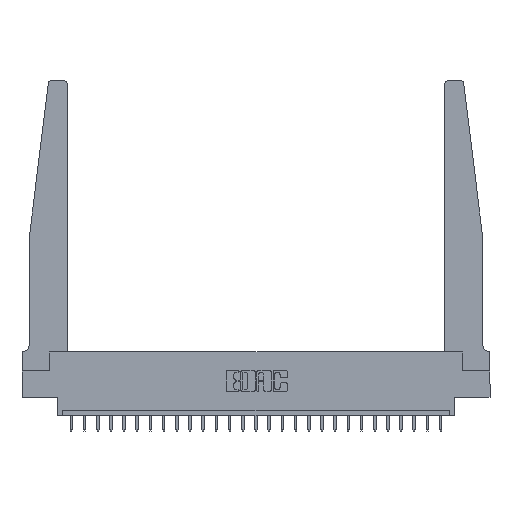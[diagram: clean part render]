
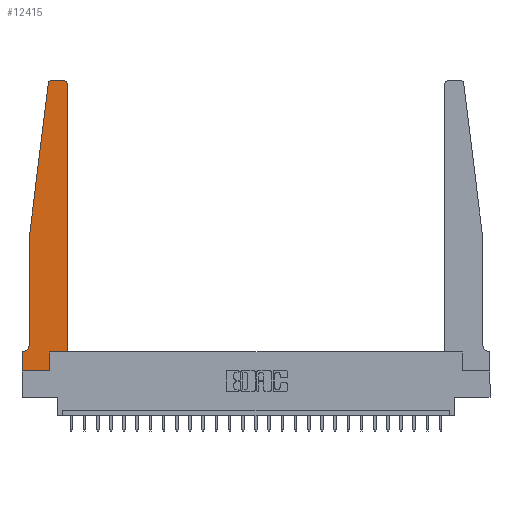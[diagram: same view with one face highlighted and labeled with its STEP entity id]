
A CAD part, top view. The second image highlights one B-rep face of the part: STEP entity #12415.
In plain terms, the highlighted planar face has unit normal (0, 0, 1).
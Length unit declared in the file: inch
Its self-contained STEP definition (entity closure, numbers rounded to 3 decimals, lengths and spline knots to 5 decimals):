
#265 = CARTESIAN_POINT ( 'NONE',  ( 0.27653, 2.75, 0.37 ) ) ;
#551 = VERTEX_POINT ( 'NONE', #13449 ) ;
#1065 = CIRCLE ( 'NONE', #18490, 0.03 ) ;
#1085 = EDGE_CURVE ( 'NONE', #22084, #10437, #18682, .T. ) ;
#1307 = CARTESIAN_POINT ( 'NONE',  ( 0.065, 1.25, 0.37 ) ) ;
#1937 = ORIENTED_EDGE ( 'NONE', *, *, #7434, .T. ) ;
#2708 = FACE_OUTER_BOUND ( 'NONE', #15776, .T. ) ;
#2877 = VERTEX_POINT ( 'NONE', #5473 ) ;
#2949 = VERTEX_POINT ( 'NONE', #265 ) ;
#3255 = ORIENTED_EDGE ( 'NONE', *, *, #1085, .T. ) ;
#3620 = DIRECTION ( 'NONE',  ( 1., 0., 0. ) ) ;
#3899 = DIRECTION ( 'NONE',  ( -1., 0., 0. ) ) ;
#4337 = ORIENTED_EDGE ( 'NONE', *, *, #23094, .T. ) ;
#4642 = VECTOR ( 'NONE', #22095, 39.37008 ) ;
#4856 = CARTESIAN_POINT ( 'NONE',  ( 0., 0.1875, 0.37 ) ) ;
#4949 = VECTOR ( 'NONE', #19105, 39.37008 ) ;
#5077 = LINE ( 'NONE', #8885, #6246 ) ;
#5325 = ORIENTED_EDGE ( 'NONE', *, *, #13525, .T. ) ;
#5349 = EDGE_CURVE ( 'NONE', #2949, #21349, #1065, .T. ) ;
#5393 = CARTESIAN_POINT ( 'NONE',  ( 0.27653, 2.72, 0.37 ) ) ;
#5473 = CARTESIAN_POINT ( 'NONE',  ( 0.015, 0.1875, 0.37 ) ) ;
#5707 = VECTOR ( 'NONE', #24729, 39.37008 ) ;
#5776 = CARTESIAN_POINT ( 'NONE',  ( 0.065, 1.25, 0.37 ) ) ;
#5852 = VERTEX_POINT ( 'NONE', #11840 ) ;
#6006 = ORIENTED_EDGE ( 'NONE', *, *, #8162, .T. ) ;
#6246 = VECTOR ( 'NONE', #9011, 39.37008 ) ;
#6573 = VECTOR ( 'NONE', #14024, 39.37008 ) ;
#7024 = CIRCLE ( 'NONE', #11896, 0.05 ) ;
#7296 = DIRECTION ( 'NONE',  ( 0., 0., 1. ) ) ;
#7434 = EDGE_CURVE ( 'NONE', #551, #16910, #12956, .T. ) ;
#7907 = CIRCLE ( 'NONE', #13582, 0.03 ) ;
#7951 = LINE ( 'NONE', #21270, #11808 ) ;
#8162 = EDGE_CURVE ( 'NONE', #11863, #20647, #7907, .T. ) ;
#8324 = CARTESIAN_POINT ( 'NONE',  ( 0.425, 2.72, 0.37 ) ) ;
#8431 = VECTOR ( 'NONE', #19429, 39.37008 ) ;
#8752 = CARTESIAN_POINT ( 'NONE',  ( 0.425, 0.18, 0.37 ) ) ;
#8885 = CARTESIAN_POINT ( 'NONE',  ( 0.25, 2.75, 0.37 ) ) ;
#9011 = DIRECTION ( 'NONE',  ( -1., 0., 0. ) ) ;
#9510 = CARTESIAN_POINT ( 'NONE',  ( 0.425, 0.18, 0.37 ) ) ;
#9740 = CARTESIAN_POINT ( 'NONE',  ( 0.395, 2.75, 0.37 ) ) ;
#9754 = DIRECTION ( 'NONE',  ( 0., 0., -1. ) ) ;
#9879 = CARTESIAN_POINT ( 'NONE',  ( 0.015, 0.2375, 0.37 ) ) ;
#10157 = CARTESIAN_POINT ( 'NONE',  ( 0.425, 0.18, 0.37 ) ) ;
#10437 = VERTEX_POINT ( 'NONE', #24971 ) ;
#10454 = DIRECTION ( 'NONE',  ( 0., 0., 1. ) ) ;
#10703 = PLANE ( 'NONE',  #14245 ) ;
#11179 = ORIENTED_EDGE ( 'NONE', *, *, #24212, .T. ) ;
#11567 = ORIENTED_EDGE ( 'NONE', *, *, #13350, .T. ) ;
#11808 = VECTOR ( 'NONE', #3899, 39.37008 ) ;
#11840 = CARTESIAN_POINT ( 'NONE',  ( 0., 0.1875, 0.37 ) ) ;
#11863 = VERTEX_POINT ( 'NONE', #8324 ) ;
#11896 = AXIS2_PLACEMENT_3D ( 'NONE', #9879, #9754, #17480 ) ;
#12007 = LINE ( 'NONE', #5776, #6573 ) ;
#12317 = VERTEX_POINT ( 'NONE', #16888 ) ;
#12415 = ADVANCED_FACE ( 'NONE', ( #2708 ), #10703, .T. ) ;
#12926 = LINE ( 'NONE', #9510, #5707 ) ;
#12956 = LINE ( 'NONE', #10157, #8431 ) ;
#13350 = EDGE_CURVE ( 'NONE', #5852, #12317, #22928, .T. ) ;
#13364 = LINE ( 'NONE', #17874, #24328 ) ;
#13449 = CARTESIAN_POINT ( 'NONE',  ( 0.2605, 0.18, 0.37 ) ) ;
#13525 = EDGE_CURVE ( 'NONE', #21349, #22084, #12007, .T. ) ;
#13582 = AXIS2_PLACEMENT_3D ( 'NONE', #23032, #23147, #24799 ) ;
#13706 = ORIENTED_EDGE ( 'NONE', *, *, #18744, .T. ) ;
#13967 = DIRECTION ( 'NONE',  ( 1., 0., 0. ) ) ;
#14024 = DIRECTION ( 'NONE',  ( -0.122, -0.992, 0. ) ) ;
#14245 = AXIS2_PLACEMENT_3D ( 'NONE', #4856, #10454, #14252 ) ;
#14252 = DIRECTION ( 'NONE',  ( 1., 0., 0. ) ) ;
#14548 = CARTESIAN_POINT ( 'NONE',  ( 0.065, 1.25, 0.37 ) ) ;
#14566 = ORIENTED_EDGE ( 'NONE', *, *, #17756, .T. ) ;
#14873 = LINE ( 'NONE', #16629, #4642 ) ;
#15776 = EDGE_LOOP ( 'NONE', ( #11179, #19311, #5325, #3255, #4337, #13706, #11567, #24006, #14566, #1937, #22164, #6006 ) ) ;
#16629 = CARTESIAN_POINT ( 'NONE',  ( 0.2605, 0.18, 0.37 ) ) ;
#16654 = DIRECTION ( 'NONE',  ( 0., -1., 0. ) ) ;
#16888 = CARTESIAN_POINT ( 'NONE',  ( 0., 0., 0.37 ) ) ;
#16910 = VERTEX_POINT ( 'NONE', #8752 ) ;
#17207 = CARTESIAN_POINT ( 'NONE',  ( 0., 0., 0.37 ) ) ;
#17480 = DIRECTION ( 'NONE',  ( -1., 0., 0. ) ) ;
#17756 = EDGE_CURVE ( 'NONE', #21079, #551, #14873, .T. ) ;
#17874 = CARTESIAN_POINT ( 'NONE',  ( 0., 0., 0.37 ) ) ;
#18178 = EDGE_CURVE ( 'NONE', #16910, #11863, #12926, .T. ) ;
#18490 = AXIS2_PLACEMENT_3D ( 'NONE', #5393, #7296, #3620 ) ;
#18682 = LINE ( 'NONE', #1307, #19657 ) ;
#18744 = EDGE_CURVE ( 'NONE', #2877, #5852, #7951, .T. ) ;
#18922 = CARTESIAN_POINT ( 'NONE',  ( 0.24675, 2.72367, 0.37 ) ) ;
#19105 = DIRECTION ( 'NONE',  ( 0., -1., 0. ) ) ;
#19229 = EDGE_CURVE ( 'NONE', #12317, #21079, #13364, .T. ) ;
#19311 = ORIENTED_EDGE ( 'NONE', *, *, #5349, .T. ) ;
#19429 = DIRECTION ( 'NONE',  ( 1., 0., 0. ) ) ;
#19657 = VECTOR ( 'NONE', #16654, 39.37008 ) ;
#20647 = VERTEX_POINT ( 'NONE', #9740 ) ;
#20890 = CARTESIAN_POINT ( 'NONE',  ( 0.2605, 0., 0.37 ) ) ;
#21079 = VERTEX_POINT ( 'NONE', #20890 ) ;
#21270 = CARTESIAN_POINT ( 'NONE',  ( 0.065, 0.1875, 0.37 ) ) ;
#21349 = VERTEX_POINT ( 'NONE', #18922 ) ;
#22084 = VERTEX_POINT ( 'NONE', #14548 ) ;
#22095 = DIRECTION ( 'NONE',  ( 0., 1., 0. ) ) ;
#22164 = ORIENTED_EDGE ( 'NONE', *, *, #18178, .T. ) ;
#22928 = LINE ( 'NONE', #17207, #4949 ) ;
#23032 = CARTESIAN_POINT ( 'NONE',  ( 0.395, 2.72, 0.37 ) ) ;
#23094 = EDGE_CURVE ( 'NONE', #10437, #2877, #7024, .T. ) ;
#23147 = DIRECTION ( 'NONE',  ( 0., 0., 1. ) ) ;
#24006 = ORIENTED_EDGE ( 'NONE', *, *, #19229, .T. ) ;
#24212 = EDGE_CURVE ( 'NONE', #20647, #2949, #5077, .T. ) ;
#24328 = VECTOR ( 'NONE', #13967, 39.37008 ) ;
#24729 = DIRECTION ( 'NONE',  ( 0., 1., 0. ) ) ;
#24799 = DIRECTION ( 'NONE',  ( 1., 0., 0. ) ) ;
#24971 = CARTESIAN_POINT ( 'NONE',  ( 0.065, 0.2375, 0.37 ) ) ;
